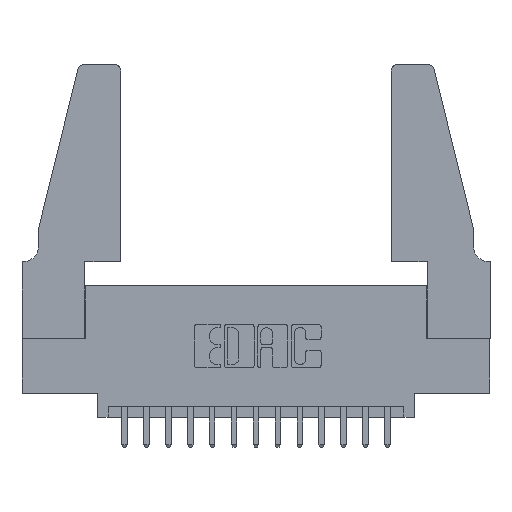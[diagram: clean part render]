
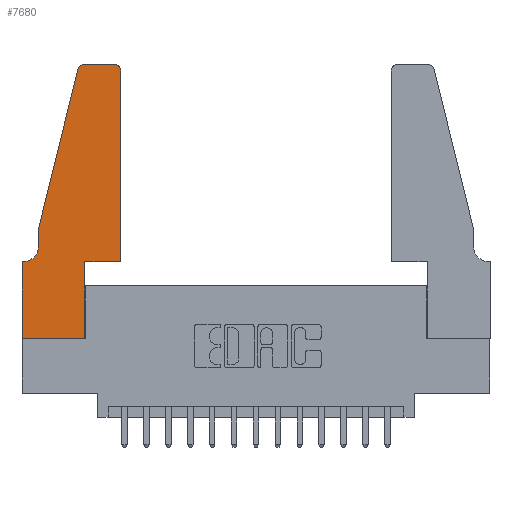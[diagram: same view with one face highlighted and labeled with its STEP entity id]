
A CAD part, top view. The second image highlights one B-rep face of the part: STEP entity #7680.
In plain terms, the highlighted planar face has unit normal (0, 0, 1).
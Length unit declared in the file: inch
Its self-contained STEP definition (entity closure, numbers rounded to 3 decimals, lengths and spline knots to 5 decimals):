
#41 = CARTESIAN_POINT ( 'NONE',  ( 0., 0.35, 0.37 ) ) ;
#302 = EDGE_CURVE ( 'NONE', #12655, #7788, #13614, .T. ) ;
#777 = VERTEX_POINT ( 'NONE', #7499 ) ;
#806 = AXIS2_PLACEMENT_3D ( 'NONE', #9539, #10702, #14544 ) ;
#1040 = FACE_OUTER_BOUND ( 'NONE', #7593, .T. ) ;
#1045 = EDGE_CURVE ( 'NONE', #7777, #3330, #9012, .T. ) ;
#1066 = ORIENTED_EDGE ( 'NONE', *, *, #5611, .T. ) ;
#1130 = AXIS2_PLACEMENT_3D ( 'NONE', #2365, #6378, #7621 ) ;
#1173 = ORIENTED_EDGE ( 'NONE', *, *, #6268, .T. ) ;
#1204 = DIRECTION ( 'NONE',  ( -1., 0., 0. ) ) ;
#1205 = CARTESIAN_POINT ( 'NONE',  ( 0.4505, 1.22, 0.37 ) ) ;
#1312 = CARTESIAN_POINT ( 'NONE',  ( 0.0755, 0.35, 0.37 ) ) ;
#1738 = EDGE_CURVE ( 'NONE', #14149, #777, #5761, .T. ) ;
#1855 = CARTESIAN_POINT ( 'NONE',  ( 0.0755, 0.5, 0.37 ) ) ;
#1987 = VERTEX_POINT ( 'NONE', #15739 ) ;
#2077 = CARTESIAN_POINT ( 'NONE',  ( 0., 0., 0.37 ) ) ;
#2365 = CARTESIAN_POINT ( 'NONE',  ( 0.0055, 0.42, 0.37 ) ) ;
#2393 = CARTESIAN_POINT ( 'NONE',  ( 0., 0.35, 0.37 ) ) ;
#2483 = CARTESIAN_POINT ( 'NONE',  ( 0.0755, 0.5, 0.37 ) ) ;
#2670 = CARTESIAN_POINT ( 'NONE',  ( 0.4505, 0.35, 0.37 ) ) ;
#2994 = CARTESIAN_POINT ( 'NONE',  ( 0.2865, 0., 0.37 ) ) ;
#3015 = DIRECTION ( 'NONE',  ( 0., -1., 0. ) ) ;
#3138 = AXIS2_PLACEMENT_3D ( 'NONE', #14110, #5136, #15214 ) ;
#3278 = VECTOR ( 'NONE', #12025, 39.37008 ) ;
#3330 = VERTEX_POINT ( 'NONE', #1205 ) ;
#3505 = EDGE_CURVE ( 'NONE', #777, #11695, #6495, .T. ) ;
#4217 = CARTESIAN_POINT ( 'NONE',  ( 0.2865, 0.35, 0.37 ) ) ;
#4314 = LINE ( 'NONE', #14380, #5531 ) ;
#4466 = LINE ( 'NONE', #5532, #15944 ) ;
#4743 = VERTEX_POINT ( 'NONE', #2077 ) ;
#4783 = ORIENTED_EDGE ( 'NONE', *, *, #15869, .T. ) ;
#4793 = ORIENTED_EDGE ( 'NONE', *, *, #302, .T. ) ;
#4956 = DIRECTION ( 'NONE',  ( 0., 0., 1. ) ) ;
#5136 = DIRECTION ( 'NONE',  ( 0., 0., 1. ) ) ;
#5198 = VERTEX_POINT ( 'NONE', #4217 ) ;
#5290 = ORIENTED_EDGE ( 'NONE', *, *, #13462, .T. ) ;
#5531 = VECTOR ( 'NONE', #11676, 39.37008 ) ;
#5532 = CARTESIAN_POINT ( 'NONE',  ( 0., 0., 0.37 ) ) ;
#5611 = EDGE_CURVE ( 'NONE', #12474, #12655, #8045, .T. ) ;
#5735 = CARTESIAN_POINT ( 'NONE',  ( 0.2605, 1.25, 0.37 ) ) ;
#5741 = VECTOR ( 'NONE', #7610, 39.37008 ) ;
#5761 = CIRCLE ( 'NONE', #3138, 0.03 ) ;
#6268 = EDGE_CURVE ( 'NONE', #5198, #7777, #13399, .T. ) ;
#6378 = DIRECTION ( 'NONE',  ( 0., 0., -1. ) ) ;
#6495 = LINE ( 'NONE', #1855, #8817 ) ;
#7484 = LINE ( 'NONE', #5735, #8062 ) ;
#7499 = CARTESIAN_POINT ( 'NONE',  ( 0.25487, 1.22718, 0.37 ) ) ;
#7593 = EDGE_LOOP ( 'NONE', ( #5290, #15801, #12844, #4783, #1066, #4793, #11387, #8610, #7734, #1173, #12422, #14426 ) ) ;
#7610 = DIRECTION ( 'NONE',  ( 1., 0., 0. ) ) ;
#7621 = DIRECTION ( 'NONE',  ( -1., 0., 0. ) ) ;
#7680 = ADVANCED_FACE ( 'NONE', ( #1040 ), #15036, .T. ) ;
#7734 = ORIENTED_EDGE ( 'NONE', *, *, #13372, .T. ) ;
#7777 = VERTEX_POINT ( 'NONE', #2670 ) ;
#7788 = VERTEX_POINT ( 'NONE', #41 ) ;
#8025 = CARTESIAN_POINT ( 'NONE',  ( 0.4505, 0.35, 0.37 ) ) ;
#8045 = CIRCLE ( 'NONE', #1130, 0.07 ) ;
#8062 = VECTOR ( 'NONE', #13327, 39.37008 ) ;
#8610 = ORIENTED_EDGE ( 'NONE', *, *, #9961, .T. ) ;
#8817 = VECTOR ( 'NONE', #14352, 39.37008 ) ;
#9012 = LINE ( 'NONE', #8025, #3278 ) ;
#9076 = LINE ( 'NONE', #12639, #5741 ) ;
#9088 = EDGE_CURVE ( 'NONE', #3330, #1987, #13283, .T. ) ;
#9539 = CARTESIAN_POINT ( 'NONE',  ( 0.4205, 1.22, 0.37 ) ) ;
#9961 = EDGE_CURVE ( 'NONE', #4743, #14127, #9076, .T. ) ;
#10424 = VECTOR ( 'NONE', #13184, 39.37008 ) ;
#10702 = DIRECTION ( 'NONE',  ( 0., 0., 1. ) ) ;
#10746 = CARTESIAN_POINT ( 'NONE',  ( 0.0055, 0.35, 0.37 ) ) ;
#11324 = CARTESIAN_POINT ( 'NONE',  ( 0.0755, 0.42, 0.37 ) ) ;
#11387 = ORIENTED_EDGE ( 'NONE', *, *, #15160, .T. ) ;
#11676 = DIRECTION ( 'NONE',  ( 0., 1., 0. ) ) ;
#11695 = VERTEX_POINT ( 'NONE', #2483 ) ;
#12025 = DIRECTION ( 'NONE',  ( 0., 1., 0. ) ) ;
#12422 = ORIENTED_EDGE ( 'NONE', *, *, #1045, .T. ) ;
#12474 = VERTEX_POINT ( 'NONE', #11324 ) ;
#12566 = DIRECTION ( 'NONE',  ( 1., 0., 0. ) ) ;
#12639 = CARTESIAN_POINT ( 'NONE',  ( 0., 0., 0.37 ) ) ;
#12655 = VERTEX_POINT ( 'NONE', #10746 ) ;
#12844 = ORIENTED_EDGE ( 'NONE', *, *, #3505, .T. ) ;
#12987 = VECTOR ( 'NONE', #13845, 39.37008 ) ;
#13184 = DIRECTION ( 'NONE',  ( 1., 0., 0. ) ) ;
#13283 = CIRCLE ( 'NONE', #806, 0.03 ) ;
#13327 = DIRECTION ( 'NONE',  ( -1., 0., 0. ) ) ;
#13372 = EDGE_CURVE ( 'NONE', #14127, #5198, #4314, .T. ) ;
#13399 = LINE ( 'NONE', #15779, #10424 ) ;
#13462 = EDGE_CURVE ( 'NONE', #1987, #14149, #7484, .T. ) ;
#13614 = LINE ( 'NONE', #1312, #14816 ) ;
#13787 = CARTESIAN_POINT ( 'NONE',  ( 0.0755, 0.5, 0.37 ) ) ;
#13845 = DIRECTION ( 'NONE',  ( 0., -1., 0. ) ) ;
#14110 = CARTESIAN_POINT ( 'NONE',  ( 0.284, 1.22, 0.37 ) ) ;
#14127 = VERTEX_POINT ( 'NONE', #2994 ) ;
#14149 = VERTEX_POINT ( 'NONE', #15776 ) ;
#14352 = DIRECTION ( 'NONE',  ( -0.239, -0.971, 0. ) ) ;
#14380 = CARTESIAN_POINT ( 'NONE',  ( 0.2865, 0.35, 0.37 ) ) ;
#14426 = ORIENTED_EDGE ( 'NONE', *, *, #9088, .T. ) ;
#14544 = DIRECTION ( 'NONE',  ( 1., 0., 0. ) ) ;
#14816 = VECTOR ( 'NONE', #1204, 39.37008 ) ;
#15036 = PLANE ( 'NONE',  #15719 ) ;
#15160 = EDGE_CURVE ( 'NONE', #7788, #4743, #4466, .T. ) ;
#15214 = DIRECTION ( 'NONE',  ( 1., 0., 0. ) ) ;
#15567 = LINE ( 'NONE', #13787, #12987 ) ;
#15719 = AXIS2_PLACEMENT_3D ( 'NONE', #2393, #4956, #12566 ) ;
#15739 = CARTESIAN_POINT ( 'NONE',  ( 0.4205, 1.25, 0.37 ) ) ;
#15776 = CARTESIAN_POINT ( 'NONE',  ( 0.284, 1.25, 0.37 ) ) ;
#15779 = CARTESIAN_POINT ( 'NONE',  ( 0.4505, 0.35, 0.37 ) ) ;
#15801 = ORIENTED_EDGE ( 'NONE', *, *, #1738, .T. ) ;
#15869 = EDGE_CURVE ( 'NONE', #11695, #12474, #15567, .T. ) ;
#15944 = VECTOR ( 'NONE', #3015, 39.37008 ) ;
